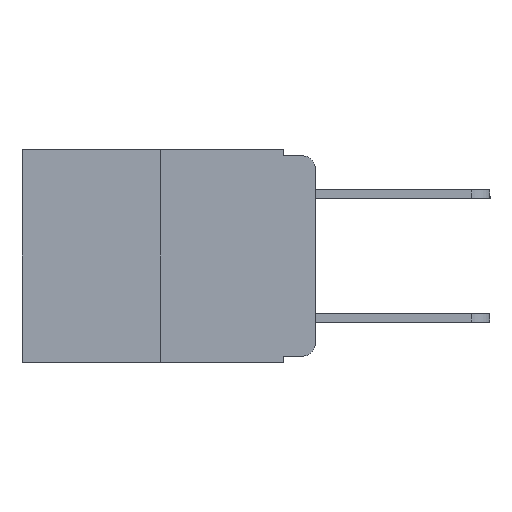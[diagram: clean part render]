
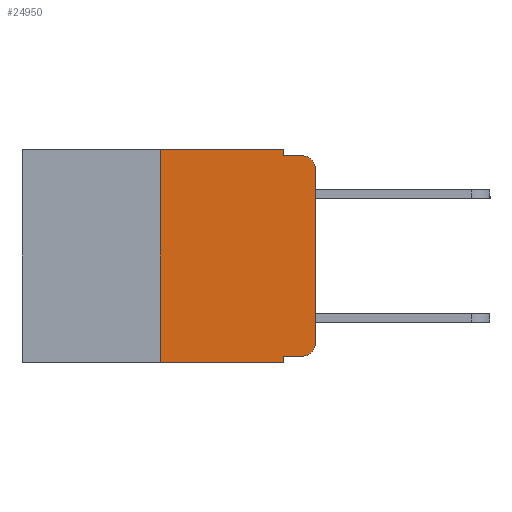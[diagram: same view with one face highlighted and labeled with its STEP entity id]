
A CAD part, left-side view. The second image highlights one B-rep face of the part: STEP entity #24950.
In plain terms, the highlighted planar face has unit normal (-1, 0, 0).
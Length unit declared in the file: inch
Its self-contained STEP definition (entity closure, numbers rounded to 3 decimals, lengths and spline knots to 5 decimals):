
#13 = LINE ( 'NONE', #18569, #4728 ) ;
#32 = VECTOR ( 'NONE', #5849, 39.37008 ) ;
#518 = AXIS2_PLACEMENT_3D ( 'NONE', #11565, #24925, #13481 ) ;
#778 = DIRECTION ( 'NONE',  ( -1., 0., 0. ) ) ;
#987 = ORIENTED_EDGE ( 'NONE', *, *, #4104, .F. ) ;
#1104 = DIRECTION ( 'NONE',  ( 0., 0., 1. ) ) ;
#1123 = EDGE_CURVE ( 'NONE', #22573, #15393, #13, .T. ) ;
#1435 = CARTESIAN_POINT ( 'NONE',  ( 0., 0.473, 0. ) ) ;
#1870 = ORIENTED_EDGE ( 'NONE', *, *, #20662, .T. ) ;
#2758 = ORIENTED_EDGE ( 'NONE', *, *, #7441, .T. ) ;
#4037 = CARTESIAN_POINT ( 'NONE',  ( 0., 0.25, -0.343 ) ) ;
#4104 = EDGE_CURVE ( 'NONE', #7014, #22573, #13029, .T. ) ;
#4141 = CARTESIAN_POINT ( 'NONE',  ( 0., 0.02, -0.333 ) ) ;
#4367 = LINE ( 'NONE', #24228, #19188 ) ;
#4728 = VECTOR ( 'NONE', #22403, 39.37008 ) ;
#4985 = VECTOR ( 'NONE', #13557, 39.37008 ) ;
#5615 = LINE ( 'NONE', #7762, #4985 ) ;
#5849 = DIRECTION ( 'NONE',  ( 0., 0., 1. ) ) ;
#5855 = CARTESIAN_POINT ( 'NONE',  ( 0., 0.051, -0.333 ) ) ;
#5865 = CARTESIAN_POINT ( 'NONE',  ( 0., 0.051, -0.343 ) ) ;
#6494 = EDGE_CURVE ( 'NONE', #19091, #7014, #21877, .T. ) ;
#6855 = CIRCLE ( 'NONE', #518, 0.02 ) ;
#7014 = VERTEX_POINT ( 'NONE', #21871 ) ;
#7165 = AXIS2_PLACEMENT_3D ( 'NONE', #9646, #19288, #7774 ) ;
#7189 = ORIENTED_EDGE ( 'NONE', *, *, #24943, .T. ) ;
#7441 = EDGE_CURVE ( 'NONE', #19091, #22235, #5615, .T. ) ;
#7587 = AXIS2_PLACEMENT_3D ( 'NONE', #12512, #778, #14434 ) ;
#7762 = CARTESIAN_POINT ( 'NONE',  ( 0., 0.473, -0.343 ) ) ;
#7774 = DIRECTION ( 'NONE',  ( 0., 0., -1. ) ) ;
#7792 = EDGE_CURVE ( 'NONE', #15513, #22235, #12551, .T. ) ;
#7823 = DIRECTION ( 'NONE',  ( 0., -1., 0. ) ) ;
#7988 = LINE ( 'NONE', #5855, #17575 ) ;
#8478 = ORIENTED_EDGE ( 'NONE', *, *, #1123, .F. ) ;
#9646 = CARTESIAN_POINT ( 'NONE',  ( 0., 0.473, 0. ) ) ;
#10000 = ORIENTED_EDGE ( 'NONE', *, *, #19890, .F. ) ;
#10554 = LINE ( 'NONE', #24965, #32 ) ;
#10869 = EDGE_CURVE ( 'NONE', #16974, #11025, #10554, .T. ) ;
#11025 = VERTEX_POINT ( 'NONE', #21666 ) ;
#11565 = CARTESIAN_POINT ( 'NONE',  ( 0., 0.02, -0.03 ) ) ;
#12512 = CARTESIAN_POINT ( 'NONE',  ( 0., 0.02, -0.313 ) ) ;
#12551 = LINE ( 'NONE', #16450, #22142 ) ;
#13029 = LINE ( 'NONE', #1435, #22615 ) ;
#13481 = DIRECTION ( 'NONE',  ( 0., 0., -1. ) ) ;
#13557 = DIRECTION ( 'NONE',  ( 0., -1., 0. ) ) ;
#14137 = ORIENTED_EDGE ( 'NONE', *, *, #10869, .T. ) ;
#14243 = EDGE_CURVE ( 'NONE', #15513, #23283, #7988, .T. ) ;
#14434 = DIRECTION ( 'NONE',  ( 0., 0., -1. ) ) ;
#14989 = ORIENTED_EDGE ( 'NONE', *, *, #14243, .T. ) ;
#15161 = DIRECTION ( 'NONE',  ( 0., -1., 0. ) ) ;
#15172 = CARTESIAN_POINT ( 'NONE',  ( 0., 0.051, -0.01 ) ) ;
#15393 = VERTEX_POINT ( 'NONE', #15172 ) ;
#15513 = VERTEX_POINT ( 'NONE', #23214 ) ;
#15869 = CARTESIAN_POINT ( 'NONE',  ( 0., 0.02, -0.01 ) ) ;
#16153 = VECTOR ( 'NONE', #1104, 39.37008 ) ;
#16192 = EDGE_LOOP ( 'NONE', ( #14137, #7189, #10000, #8478, #987, #17118, #2758, #17415, #14989, #1870 ) ) ;
#16450 = CARTESIAN_POINT ( 'NONE',  ( 0., 0.051, 0. ) ) ;
#16974 = VERTEX_POINT ( 'NONE', #24076 ) ;
#17067 = FACE_OUTER_BOUND ( 'NONE', #16192, .T. ) ;
#17118 = ORIENTED_EDGE ( 'NONE', *, *, #6494, .F. ) ;
#17325 = PLANE ( 'NONE',  #7165 ) ;
#17415 = ORIENTED_EDGE ( 'NONE', *, *, #7792, .F. ) ;
#17575 = VECTOR ( 'NONE', #7823, 39.37008 ) ;
#18492 = DIRECTION ( 'NONE',  ( 0., 0., -1. ) ) ;
#18554 = CARTESIAN_POINT ( 'NONE',  ( 0., 0.25, 0. ) ) ;
#18569 = CARTESIAN_POINT ( 'NONE',  ( 0., 0.051, 0. ) ) ;
#19091 = VERTEX_POINT ( 'NONE', #4037 ) ;
#19187 = VERTEX_POINT ( 'NONE', #15869 ) ;
#19188 = VECTOR ( 'NONE', #22153, 39.37008 ) ;
#19288 = DIRECTION ( 'NONE',  ( 1., 0., 0. ) ) ;
#19890 = EDGE_CURVE ( 'NONE', #15393, #19187, #4367, .T. ) ;
#20662 = EDGE_CURVE ( 'NONE', #23283, #16974, #22131, .T. ) ;
#21666 = CARTESIAN_POINT ( 'NONE',  ( 0., 0., -0.03 ) ) ;
#21871 = CARTESIAN_POINT ( 'NONE',  ( 0., 0.25, 0. ) ) ;
#21877 = LINE ( 'NONE', #18554, #16153 ) ;
#22131 = CIRCLE ( 'NONE', #7587, 0.02 ) ;
#22142 = VECTOR ( 'NONE', #18492, 39.37008 ) ;
#22153 = DIRECTION ( 'NONE',  ( 0., -1., 0. ) ) ;
#22235 = VERTEX_POINT ( 'NONE', #5865 ) ;
#22403 = DIRECTION ( 'NONE',  ( 0., 0., -1. ) ) ;
#22573 = VERTEX_POINT ( 'NONE', #24225 ) ;
#22615 = VECTOR ( 'NONE', #15161, 39.37008 ) ;
#23214 = CARTESIAN_POINT ( 'NONE',  ( 0., 0.051, -0.333 ) ) ;
#23283 = VERTEX_POINT ( 'NONE', #4141 ) ;
#24076 = CARTESIAN_POINT ( 'NONE',  ( 0., 0., -0.313 ) ) ;
#24225 = CARTESIAN_POINT ( 'NONE',  ( 0., 0.051, 0. ) ) ;
#24228 = CARTESIAN_POINT ( 'NONE',  ( 0., 0.051, -0.01 ) ) ;
#24925 = DIRECTION ( 'NONE',  ( -1., 0., 0. ) ) ;
#24943 = EDGE_CURVE ( 'NONE', #11025, #19187, #6855, .T. ) ;
#24950 = ADVANCED_FACE ( 'NONE', ( #17067 ), #17325, .F. ) ;
#24965 = CARTESIAN_POINT ( 'NONE',  ( 0., 0., 0. ) ) ;
